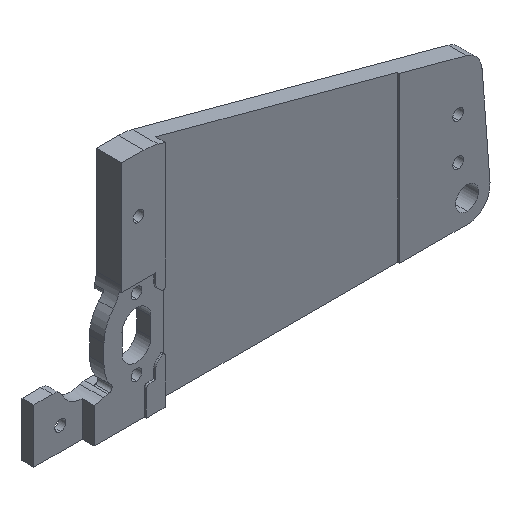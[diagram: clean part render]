
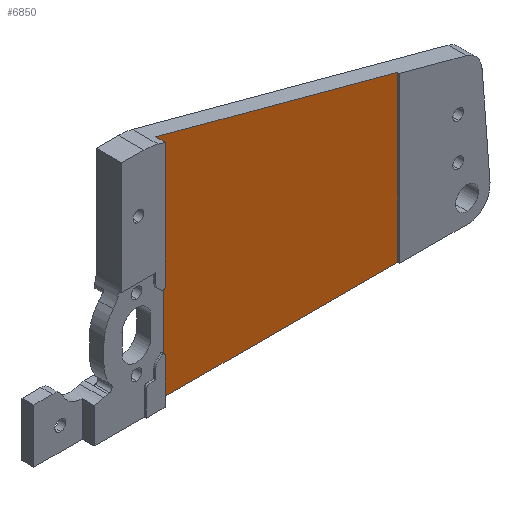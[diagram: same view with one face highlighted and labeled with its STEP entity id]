
A CAD part, isometric view. The second image highlights one B-rep face of the part: STEP entity #6850.
In plain terms, the highlighted planar face has unit normal (0, -1, 0).
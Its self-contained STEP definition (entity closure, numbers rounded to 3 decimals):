
#181 = VECTOR ( 'NONE', #3521, 1000. ) ;
#385 = ORIENTED_EDGE ( 'NONE', *, *, #6824, .T. ) ;
#442 = CARTESIAN_POINT ( 'NONE',  ( 0., 2.545, 0. ) ) ;
#493 = DIRECTION ( 'NONE',  ( 0., 0., -1. ) ) ;
#523 = CARTESIAN_POINT ( 'NONE',  ( 78.632, 2.545, -19.375 ) ) ;
#772 = DIRECTION ( 'NONE',  ( -0.966, 0., 0.26 ) ) ;
#789 = CARTESIAN_POINT ( 'NONE',  ( 77.132, 2.545, -64.364 ) ) ;
#1568 = LINE ( 'NONE', #523, #4198 ) ;
#1632 = ORIENTED_EDGE ( 'NONE', *, *, #11490, .T. ) ;
#2001 = ORIENTED_EDGE ( 'NONE', *, *, #7856, .F. ) ;
#2375 = ORIENTED_EDGE ( 'NONE', *, *, #11098, .T. ) ;
#2477 = VERTEX_POINT ( 'NONE', #10198 ) ;
#3132 = AXIS2_PLACEMENT_3D ( 'NONE', #442, #3459, #6362 ) ;
#3333 = PLANE ( 'NONE',  #3132 ) ;
#3459 = DIRECTION ( 'NONE',  ( 0., -1., 0. ) ) ;
#3521 = DIRECTION ( 'NONE',  ( 1., 0., 0. ) ) ;
#3948 = CARTESIAN_POINT ( 'NONE',  ( 77.132, 2.545, -17.55 ) ) ;
#4198 = VECTOR ( 'NONE', #772, 1000. ) ;
#4785 = VECTOR ( 'NONE', #493, 1000. ) ;
#5181 = VERTEX_POINT ( 'NONE', #9641 ) ;
#6117 = LINE ( 'NONE', #9886, #181 ) ;
#6362 = DIRECTION ( 'NONE',  ( 1., 0., 0. ) ) ;
#6824 = EDGE_CURVE ( 'NONE', #7031, #10365, #6117, .T. ) ;
#6850 = ADVANCED_FACE ( 'NONE', ( #11861 ), #3333, .T. ) ;
#7031 = VERTEX_POINT ( 'NONE', #7353 ) ;
#7353 = CARTESIAN_POINT ( 'NONE',  ( 10.432, 2.545, -64.364 ) ) ;
#7856 = EDGE_CURVE ( 'NONE', #2477, #10365, #8765, .T. ) ;
#8765 = LINE ( 'NONE', #3948, #9792 ) ;
#9641 = CARTESIAN_POINT ( 'NONE',  ( 10.432, 2.545, -1.036 ) ) ;
#9792 = VECTOR ( 'NONE', #11411, 1000. ) ;
#9886 = CARTESIAN_POINT ( 'NONE',  ( 11.932, 2.545, -64.364 ) ) ;
#10198 = CARTESIAN_POINT ( 'NONE',  ( 77.132, 2.545, -18.971 ) ) ;
#10202 = LINE ( 'NONE', #10736, #4785 ) ;
#10365 = VERTEX_POINT ( 'NONE', #789 ) ;
#10736 = CARTESIAN_POINT ( 'NONE',  ( 10.432, 2.545, 0. ) ) ;
#11098 = EDGE_CURVE ( 'NONE', #5181, #7031, #10202, .T. ) ;
#11195 = EDGE_LOOP ( 'NONE', ( #2001, #1632, #2375, #385 ) ) ;
#11411 = DIRECTION ( 'NONE',  ( 0., 0., -1. ) ) ;
#11490 = EDGE_CURVE ( 'NONE', #2477, #5181, #1568, .T. ) ;
#11861 = FACE_OUTER_BOUND ( 'NONE', #11195, .T. ) ;
